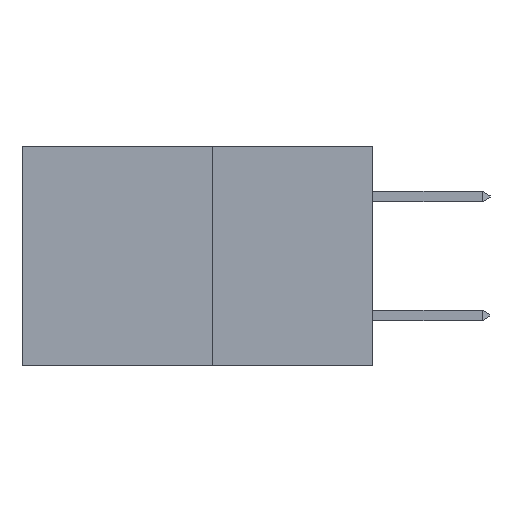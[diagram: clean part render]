
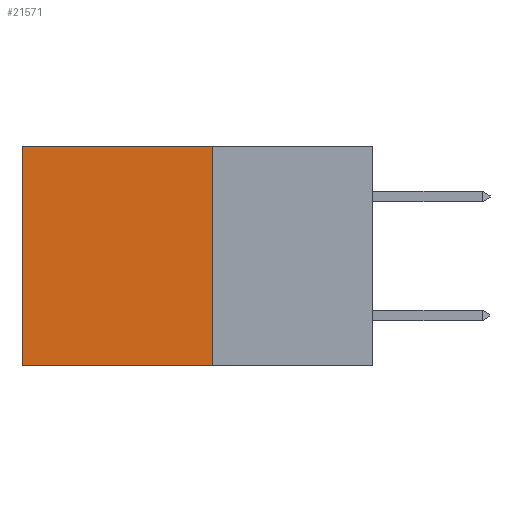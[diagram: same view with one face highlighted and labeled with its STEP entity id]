
A CAD part, left-side view. The second image highlights one B-rep face of the part: STEP entity #21571.
In plain terms, the highlighted planar face has unit normal (-1, 0, 0).
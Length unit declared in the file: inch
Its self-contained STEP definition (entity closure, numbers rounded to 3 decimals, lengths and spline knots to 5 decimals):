
#243 = CARTESIAN_POINT ( 'NONE',  ( 0.277, 0.27, -0.37 ) ) ;
#308 = EDGE_CURVE ( 'NONE', #7384, #19122, #5939, .T. ) ;
#318 = PLANE ( 'NONE',  #3744 ) ;
#1434 = DIRECTION ( 'NONE',  ( 0., 0., -1. ) ) ;
#1668 = ORIENTED_EDGE ( 'NONE', *, *, #21545, .F. ) ;
#2164 = DIRECTION ( 'NONE',  ( 1., 0., 0. ) ) ;
#2250 = VERTEX_POINT ( 'NONE', #16085 ) ;
#3074 = EDGE_CURVE ( 'NONE', #2250, #17170, #20091, .T. ) ;
#3744 = AXIS2_PLACEMENT_3D ( 'NONE', #5824, #2164, #15054 ) ;
#4114 = VECTOR ( 'NONE', #13132, 39.37008 ) ;
#5301 = ORIENTED_EDGE ( 'NONE', *, *, #8686, .T. ) ;
#5607 = CARTESIAN_POINT ( 'NONE',  ( 0.277, 0.27, 0. ) ) ;
#5824 = CARTESIAN_POINT ( 'NONE',  ( 0.277, 0.27, -0.37 ) ) ;
#5939 = LINE ( 'NONE', #5607, #20481 ) ;
#7384 = VERTEX_POINT ( 'NONE', #7509 ) ;
#7430 = CARTESIAN_POINT ( 'NONE',  ( 0.277, 0.59, -0.37 ) ) ;
#7509 = CARTESIAN_POINT ( 'NONE',  ( 0.277, 0.27, 0. ) ) ;
#8686 = EDGE_CURVE ( 'NONE', #19122, #17170, #9739, .T. ) ;
#9365 = VECTOR ( 'NONE', #22139, 39.37008 ) ;
#9739 = LINE ( 'NONE', #12584, #13950 ) ;
#12584 = CARTESIAN_POINT ( 'NONE',  ( 0.277, 0.59, -0.37 ) ) ;
#12684 = DIRECTION ( 'NONE',  ( 0., 1., 0. ) ) ;
#13132 = DIRECTION ( 'NONE',  ( 0., 0., -1. ) ) ;
#13950 = VECTOR ( 'NONE', #1434, 39.37008 ) ;
#15054 = DIRECTION ( 'NONE',  ( 0., 0., -1. ) ) ;
#16085 = CARTESIAN_POINT ( 'NONE',  ( 0.277, 0.27, -0.37 ) ) ;
#17170 = VERTEX_POINT ( 'NONE', #7430 ) ;
#17581 = LINE ( 'NONE', #243, #4114 ) ;
#18024 = ORIENTED_EDGE ( 'NONE', *, *, #3074, .F. ) ;
#19122 = VERTEX_POINT ( 'NONE', #22510 ) ;
#20091 = LINE ( 'NONE', #21052, #9365 ) ;
#20481 = VECTOR ( 'NONE', #12684, 39.37008 ) ;
#21052 = CARTESIAN_POINT ( 'NONE',  ( 0.277, 0.27, -0.37 ) ) ;
#21545 = EDGE_CURVE ( 'NONE', #7384, #2250, #17581, .T. ) ;
#21571 = ADVANCED_FACE ( 'NONE', ( #22376 ), #318, .F. ) ;
#21909 = ORIENTED_EDGE ( 'NONE', *, *, #308, .T. ) ;
#22139 = DIRECTION ( 'NONE',  ( 0., 1., 0. ) ) ;
#22340 = EDGE_LOOP ( 'NONE', ( #5301, #18024, #1668, #21909 ) ) ;
#22376 = FACE_OUTER_BOUND ( 'NONE', #22340, .T. ) ;
#22510 = CARTESIAN_POINT ( 'NONE',  ( 0.277, 0.59, 0. ) ) ;
